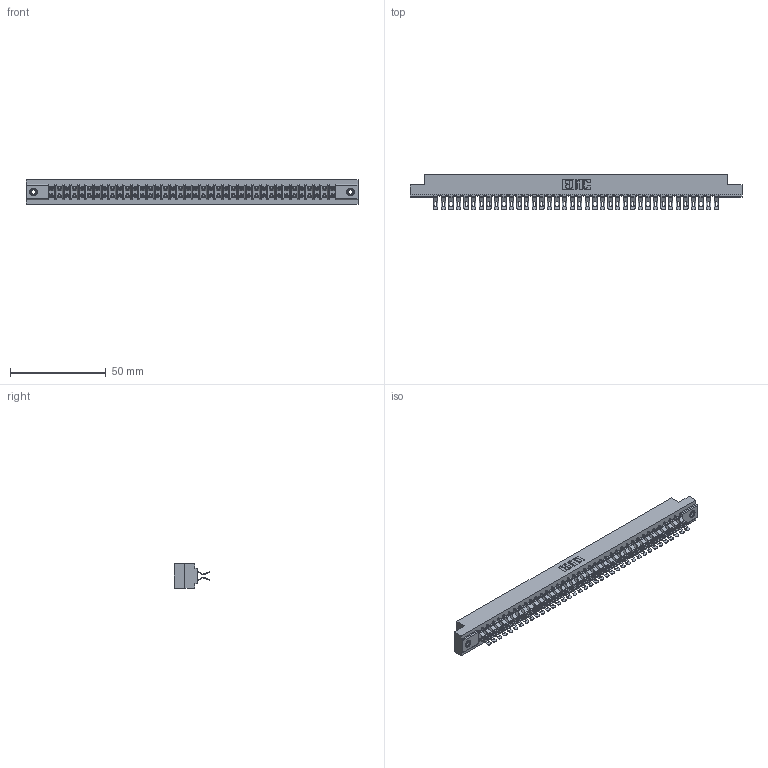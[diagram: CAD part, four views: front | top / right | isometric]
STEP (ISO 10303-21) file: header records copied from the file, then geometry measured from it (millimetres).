
FILE_DESCRIPTION (( 'STEP AP203' ), '1' );
FILE_NAME ('307-076-455-208.STEP', '2020-10-01T05:27:17', ( '' ), ( '' ), 'SwSTEP 2.0', 'SolidWorks 2020', '' );
FILE_SCHEMA (( 'CONFIG_CONTROL_DESIGN' ));
Length unit declared in the file: inch
Products named in the file (4): 345-250-001_345-250-003-102; 307-290-001_555; 307 Part_.156 Dia Mounting Holes; 307-076-455-208
Assembly tree (79 placements, depth 2):
  307-076-455-208
    307 Part_.156 Dia Mounting Holes
    307-290-001_555  x76
    345-250-001_345-250-003-102  x2
Bounding box: 173.58 x 18.75 x 12.7 mm (x, y, z)
Volume: 18650.1 mm3; surface area: 24016.2 mm2
Topology: 79 solids, 79 shells, 4853 faces, 14215 edges, 9262 vertices
Faces by surface type: plane 2686, cylinder 2073, sphere 78, cone 12, torus 4
Entity records: 36008 total; most frequent: CARTESIAN_POINT 5881, ORIENTED_EDGE 5824, DIRECTION 5778, EDGE_CURVE 2912, LINE 2220, VECTOR 2220, VERTEX_POINT 1882, AXIS2_PLACEMENT_3D 1779
